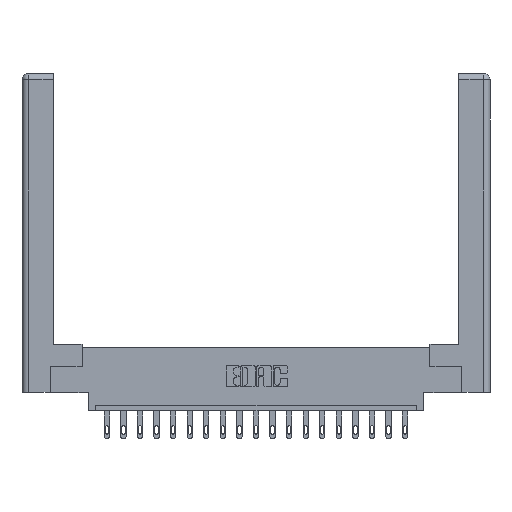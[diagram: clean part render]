
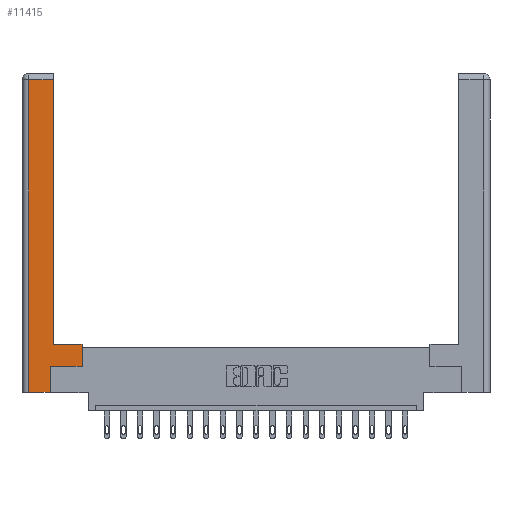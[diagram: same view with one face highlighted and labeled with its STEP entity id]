
A CAD part, top view. The second image highlights one B-rep face of the part: STEP entity #11415.
In plain terms, the highlighted planar face has unit normal (0, 0, 1).
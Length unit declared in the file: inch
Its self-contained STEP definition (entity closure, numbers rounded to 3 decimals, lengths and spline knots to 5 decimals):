
#33 = CARTESIAN_POINT ( 'NONE',  ( 0., 0., 0. ) ) ;
#190 = CARTESIAN_POINT ( 'NONE',  ( 0.565, 0.245, 0. ) ) ;
#206 = ORIENTED_EDGE ( 'NONE', *, *, #19415, .T. ) ;
#670 = VECTOR ( 'NONE', #18121, 39.37008 ) ;
#727 = CARTESIAN_POINT ( 'NONE',  ( 0.295, 3., 0. ) ) ;
#858 = LINE ( 'NONE', #727, #1349 ) ;
#1302 = ORIENTED_EDGE ( 'NONE', *, *, #18653, .T. ) ;
#1349 = VECTOR ( 'NONE', #19073, 39.37008 ) ;
#2020 = VERTEX_POINT ( 'NONE', #6029 ) ;
#2047 = VERTEX_POINT ( 'NONE', #6493 ) ;
#2608 = EDGE_CURVE ( 'NONE', #2020, #9488, #4251, .T. ) ;
#2737 = VECTOR ( 'NONE', #12227, 39.37008 ) ;
#2945 = ORIENTED_EDGE ( 'NONE', *, *, #14800, .T. ) ;
#3143 = VERTEX_POINT ( 'NONE', #10444 ) ;
#3468 = LINE ( 'NONE', #8928, #19268 ) ;
#3574 = EDGE_CURVE ( 'NONE', #7854, #3143, #10433, .T. ) ;
#3753 = CARTESIAN_POINT ( 'NONE',  ( 0.265, 0., 0. ) ) ;
#3854 = LINE ( 'NONE', #17206, #10571 ) ;
#4251 = LINE ( 'NONE', #17988, #670 ) ;
#4491 = VERTEX_POINT ( 'NONE', #16260 ) ;
#5047 = CARTESIAN_POINT ( 'NONE',  ( 0.0615, 2.94, 0. ) ) ;
#5106 = VECTOR ( 'NONE', #7682, 39.37008 ) ;
#5576 = EDGE_CURVE ( 'NONE', #4491, #8746, #13254, .T. ) ;
#5673 = CARTESIAN_POINT ( 'NONE',  ( 0.0615, 2.94, 0. ) ) ;
#6029 = CARTESIAN_POINT ( 'NONE',  ( 0.265, 0.245, 0. ) ) ;
#6045 = ORIENTED_EDGE ( 'NONE', *, *, #3574, .T. ) ;
#6306 = EDGE_CURVE ( 'NONE', #9488, #2047, #3854, .T. ) ;
#6419 = VECTOR ( 'NONE', #17646, 39.37008 ) ;
#6493 = CARTESIAN_POINT ( 'NONE',  ( 0.565, 0.45, 0. ) ) ;
#6726 = ORIENTED_EDGE ( 'NONE', *, *, #6306, .T. ) ;
#6816 = LINE ( 'NONE', #7558, #5106 ) ;
#7206 = DIRECTION ( 'NONE',  ( -1., 0., 0. ) ) ;
#7558 = CARTESIAN_POINT ( 'NONE',  ( 0.0615, 0., 0. ) ) ;
#7682 = DIRECTION ( 'NONE',  ( 0., -1., 0. ) ) ;
#7791 = CARTESIAN_POINT ( 'NONE',  ( 0.295, 0.45, 0. ) ) ;
#7854 = VERTEX_POINT ( 'NONE', #15831 ) ;
#8738 = DIRECTION ( 'NONE',  ( 0., 1., 0. ) ) ;
#8746 = VERTEX_POINT ( 'NONE', #5047 ) ;
#8928 = CARTESIAN_POINT ( 'NONE',  ( 0.265, 0.245, 0. ) ) ;
#9216 = VECTOR ( 'NONE', #7206, 39.37008 ) ;
#9462 = LINE ( 'NONE', #7791, #2737 ) ;
#9488 = VERTEX_POINT ( 'NONE', #190 ) ;
#9570 = ORIENTED_EDGE ( 'NONE', *, *, #5576, .T. ) ;
#10147 = ORIENTED_EDGE ( 'NONE', *, *, #2608, .T. ) ;
#10407 = EDGE_LOOP ( 'NONE', ( #2945, #9570, #13034, #6045, #1302, #10147, #6726, #206 ) ) ;
#10433 = LINE ( 'NONE', #3753, #6419 ) ;
#10444 = CARTESIAN_POINT ( 'NONE',  ( 0.265, 0., 0. ) ) ;
#10467 = VERTEX_POINT ( 'NONE', #17212 ) ;
#10571 = VECTOR ( 'NONE', #15678, 39.37008 ) ;
#11415 = ADVANCED_FACE ( 'NONE', ( #14530 ), #14366, .F. ) ;
#12227 = DIRECTION ( 'NONE',  ( -1., 0., 0. ) ) ;
#12252 = DIRECTION ( 'NONE',  ( -1., 0., 0. ) ) ;
#13034 = ORIENTED_EDGE ( 'NONE', *, *, #16264, .T. ) ;
#13254 = LINE ( 'NONE', #5673, #9216 ) ;
#14366 = PLANE ( 'NONE',  #15448 ) ;
#14530 = FACE_OUTER_BOUND ( 'NONE', #10407, .T. ) ;
#14800 = EDGE_CURVE ( 'NONE', #10467, #4491, #858, .T. ) ;
#15448 = AXIS2_PLACEMENT_3D ( 'NONE', #33, #15793, #12252 ) ;
#15678 = DIRECTION ( 'NONE',  ( 0., 1., 0. ) ) ;
#15793 = DIRECTION ( 'NONE',  ( 0., 0., -1. ) ) ;
#15831 = CARTESIAN_POINT ( 'NONE',  ( 0.0615, 0., 0. ) ) ;
#16260 = CARTESIAN_POINT ( 'NONE',  ( 0.295, 2.94, 0. ) ) ;
#16264 = EDGE_CURVE ( 'NONE', #8746, #7854, #6816, .T. ) ;
#17206 = CARTESIAN_POINT ( 'NONE',  ( 0.565, 0.45, 0. ) ) ;
#17212 = CARTESIAN_POINT ( 'NONE',  ( 0.295, 0.45, 0. ) ) ;
#17646 = DIRECTION ( 'NONE',  ( 1., 0., 0. ) ) ;
#17988 = CARTESIAN_POINT ( 'NONE',  ( 0.565, 0.245, 0. ) ) ;
#18121 = DIRECTION ( 'NONE',  ( 1., 0., 0. ) ) ;
#18653 = EDGE_CURVE ( 'NONE', #3143, #2020, #3468, .T. ) ;
#19073 = DIRECTION ( 'NONE',  ( 0., 1., 0. ) ) ;
#19268 = VECTOR ( 'NONE', #8738, 39.37008 ) ;
#19415 = EDGE_CURVE ( 'NONE', #2047, #10467, #9462, .T. ) ;
